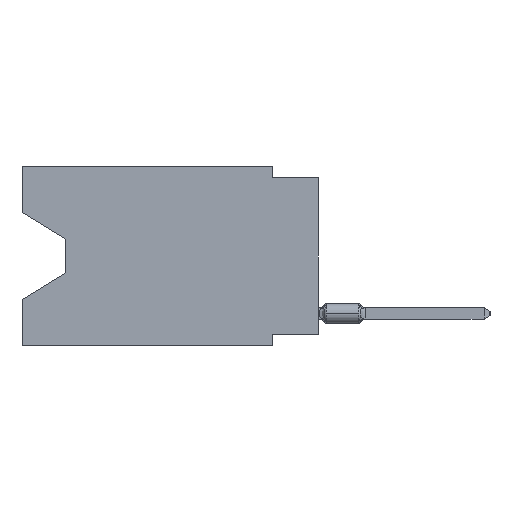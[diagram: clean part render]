
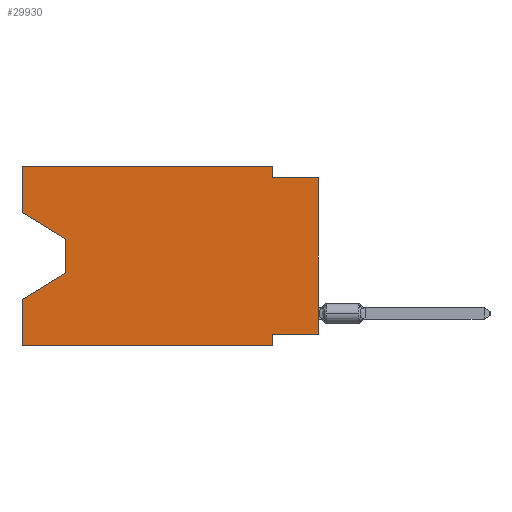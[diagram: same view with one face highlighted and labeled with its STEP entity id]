
A CAD part, left-side view. The second image highlights one B-rep face of the part: STEP entity #29930.
In plain terms, the highlighted planar face has unit normal (-1, 0, 0).
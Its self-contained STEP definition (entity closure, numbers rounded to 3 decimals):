
#198 = AXIS2_PLACEMENT_3D ( 'NONE', #23234, #68708, #79894 ) ;
#296 = CARTESIAN_POINT ( 'NONE',  ( 0., 16.383, 0. ) ) ;
#365 = EDGE_CURVE ( 'NONE', #39058, #63460, #15081, .T. ) ;
#1367 = CARTESIAN_POINT ( 'NONE',  ( 0., 2.54, -9.906 ) ) ;
#2382 = ORIENTED_EDGE ( 'NONE', *, *, #74156, .T. ) ;
#2585 = EDGE_CURVE ( 'NONE', #17016, #13637, #3218, .T. ) ;
#2686 = DIRECTION ( 'NONE',  ( 0., 0., -1. ) ) ;
#2735 = DIRECTION ( 'NONE',  ( 0., 1., 0. ) ) ;
#3218 = LINE ( 'NONE', #35933, #30935 ) ;
#5298 = EDGE_CURVE ( 'NONE', #66644, #66974, #41770, .T. ) ;
#5921 = ORIENTED_EDGE ( 'NONE', *, *, #17558, .T. ) ;
#8786 = CARTESIAN_POINT ( 'NONE',  ( 0., 13.97, -5.893 ) ) ;
#8862 = CARTESIAN_POINT ( 'NONE',  ( 0., 0., -9.271 ) ) ;
#9012 = ORIENTED_EDGE ( 'NONE', *, *, #66911, .F. ) ;
#9187 = DIRECTION ( 'NONE',  ( 0., 0., 1. ) ) ;
#11930 = VERTEX_POINT ( 'NONE', #8862 ) ;
#13053 = LINE ( 'NONE', #296, #23961 ) ;
#13637 = VERTEX_POINT ( 'NONE', #35486 ) ;
#13813 = DIRECTION ( 'NONE',  ( 0., -1., 0. ) ) ;
#14431 = CARTESIAN_POINT ( 'NONE',  ( 0., 16.383, -7.36 ) ) ;
#15081 = LINE ( 'NONE', #60123, #72743 ) ;
#15652 = VERTEX_POINT ( 'NONE', #54430 ) ;
#17016 = VERTEX_POINT ( 'NONE', #71784 ) ;
#17558 = EDGE_CURVE ( 'NONE', #11930, #15652, #61426, .T. ) ;
#21673 = ORIENTED_EDGE ( 'NONE', *, *, #32658, .F. ) ;
#22547 = ORIENTED_EDGE ( 'NONE', *, *, #61571, .F. ) ;
#22918 = DIRECTION ( 'NONE',  ( 0., 0.855, -0.519 ) ) ;
#23234 = CARTESIAN_POINT ( 'NONE',  ( 0., 16.383, 0. ) ) ;
#23533 = LINE ( 'NONE', #48616, #31505 ) ;
#23961 = VECTOR ( 'NONE', #57269, 1000. ) ;
#24686 = ORIENTED_EDGE ( 'NONE', *, *, #80056, .T. ) ;
#24771 = DIRECTION ( 'NONE',  ( 0., -1., 0. ) ) ;
#26105 = ORIENTED_EDGE ( 'NONE', *, *, #82809, .F. ) ;
#28456 = CARTESIAN_POINT ( 'NONE',  ( 0., 2.54, 0. ) ) ;
#29804 = VECTOR ( 'NONE', #71506, 1000. ) ;
#29930 = ADVANCED_FACE ( 'NONE', ( #33581 ), #42775, .F. ) ;
#30935 = VECTOR ( 'NONE', #9187, 1000. ) ;
#31505 = VECTOR ( 'NONE', #2735, 1000. ) ;
#32534 = ORIENTED_EDGE ( 'NONE', *, *, #2585, .F. ) ;
#32658 = EDGE_CURVE ( 'NONE', #38141, #15652, #64310, .T. ) ;
#33581 = FACE_OUTER_BOUND ( 'NONE', #56512, .T. ) ;
#33975 = VECTOR ( 'NONE', #2686, 1000. ) ;
#35486 = CARTESIAN_POINT ( 'NONE',  ( 0., 16.383, 0. ) ) ;
#35933 = CARTESIAN_POINT ( 'NONE',  ( 0., 16.383, 0. ) ) ;
#36388 = CARTESIAN_POINT ( 'NONE',  ( 0., 16.383, 0. ) ) ;
#36969 = VECTOR ( 'NONE', #22918, 1000. ) ;
#38141 = VERTEX_POINT ( 'NONE', #49164 ) ;
#39058 = VERTEX_POINT ( 'NONE', #43858 ) ;
#40248 = EDGE_CURVE ( 'NONE', #77994, #63460, #40882, .T. ) ;
#40882 = LINE ( 'NONE', #1367, #29804 ) ;
#41770 = LINE ( 'NONE', #73672, #33975 ) ;
#42775 = PLANE ( 'NONE',  #198 ) ;
#43858 = CARTESIAN_POINT ( 'NONE',  ( 0., 16.383, -9.906 ) ) ;
#44753 = CARTESIAN_POINT ( 'NONE',  ( 0., 0., -0.635 ) ) ;
#45118 = CARTESIAN_POINT ( 'NONE',  ( 0., 2.54, -9.271 ) ) ;
#45333 = VECTOR ( 'NONE', #24771, 1000. ) ;
#46416 = CARTESIAN_POINT ( 'NONE',  ( 0., 2.54, -9.906 ) ) ;
#46459 = LINE ( 'NONE', #47733, #83499 ) ;
#47379 = CARTESIAN_POINT ( 'NONE',  ( 0., 13.97, -4.013 ) ) ;
#47733 = CARTESIAN_POINT ( 'NONE',  ( 0., 16.383, -2.546 ) ) ;
#48008 = CARTESIAN_POINT ( 'NONE',  ( 0., 13.97, -5.893 ) ) ;
#48235 = ORIENTED_EDGE ( 'NONE', *, *, #40248, .F. ) ;
#48616 = CARTESIAN_POINT ( 'NONE',  ( 0., 0., -9.271 ) ) ;
#49086 = DIRECTION ( 'NONE',  ( 0., 0., 1. ) ) ;
#49164 = CARTESIAN_POINT ( 'NONE',  ( 0., 2.54, -0.635 ) ) ;
#49379 = EDGE_CURVE ( 'NONE', #11930, #77994, #23533, .T. ) ;
#49673 = LINE ( 'NONE', #48008, #36969 ) ;
#49980 = DIRECTION ( 'NONE',  ( 0., -1., 0. ) ) ;
#53537 = CARTESIAN_POINT ( 'NONE',  ( 0., 2.54, 0. ) ) ;
#54430 = CARTESIAN_POINT ( 'NONE',  ( 0., 0., -0.635 ) ) ;
#56512 = EDGE_LOOP ( 'NONE', ( #24686, #80333, #2382, #9012, #70804, #48235, #68657, #5921, #21673, #26105, #22547, #32534 ) ) ;
#57269 = DIRECTION ( 'NONE',  ( 0., 0., 1. ) ) ;
#57560 = VERTEX_POINT ( 'NONE', #53537 ) ;
#59514 = DIRECTION ( 'NONE',  ( 0., 0., -1. ) ) ;
#60123 = CARTESIAN_POINT ( 'NONE',  ( 0., 16.383, -9.906 ) ) ;
#60350 = LINE ( 'NONE', #28456, #66231 ) ;
#61010 = CARTESIAN_POINT ( 'NONE',  ( 0., 0., 0. ) ) ;
#61426 = LINE ( 'NONE', #61010, #72851 ) ;
#61571 = EDGE_CURVE ( 'NONE', #13637, #57560, #81835, .T. ) ;
#62200 = VERTEX_POINT ( 'NONE', #14431 ) ;
#63460 = VERTEX_POINT ( 'NONE', #46416 ) ;
#64310 = LINE ( 'NONE', #44753, #45333 ) ;
#66231 = VECTOR ( 'NONE', #59514, 1000. ) ;
#66644 = VERTEX_POINT ( 'NONE', #47379 ) ;
#66911 = EDGE_CURVE ( 'NONE', #39058, #62200, #13053, .T. ) ;
#66974 = VERTEX_POINT ( 'NONE', #8786 ) ;
#68657 = ORIENTED_EDGE ( 'NONE', *, *, #49379, .F. ) ;
#68708 = DIRECTION ( 'NONE',  ( 1., 0., 0. ) ) ;
#70804 = ORIENTED_EDGE ( 'NONE', *, *, #365, .T. ) ;
#71506 = DIRECTION ( 'NONE',  ( 0., 0., -1. ) ) ;
#71784 = CARTESIAN_POINT ( 'NONE',  ( 0., 16.383, -2.546 ) ) ;
#72096 = VECTOR ( 'NONE', #49980, 1000. ) ;
#72743 = VECTOR ( 'NONE', #13813, 1000. ) ;
#72851 = VECTOR ( 'NONE', #49086, 1000. ) ;
#73672 = CARTESIAN_POINT ( 'NONE',  ( 0., 13.97, -4.013 ) ) ;
#74156 = EDGE_CURVE ( 'NONE', #66974, #62200, #49673, .T. ) ;
#77994 = VERTEX_POINT ( 'NONE', #45118 ) ;
#79183 = DIRECTION ( 'NONE',  ( 0., -0.855, -0.519 ) ) ;
#79894 = DIRECTION ( 'NONE',  ( 0., 0., -1. ) ) ;
#80056 = EDGE_CURVE ( 'NONE', #17016, #66644, #46459, .T. ) ;
#80333 = ORIENTED_EDGE ( 'NONE', *, *, #5298, .T. ) ;
#81835 = LINE ( 'NONE', #36388, #72096 ) ;
#82809 = EDGE_CURVE ( 'NONE', #57560, #38141, #60350, .T. ) ;
#83499 = VECTOR ( 'NONE', #79183, 1000. ) ;
